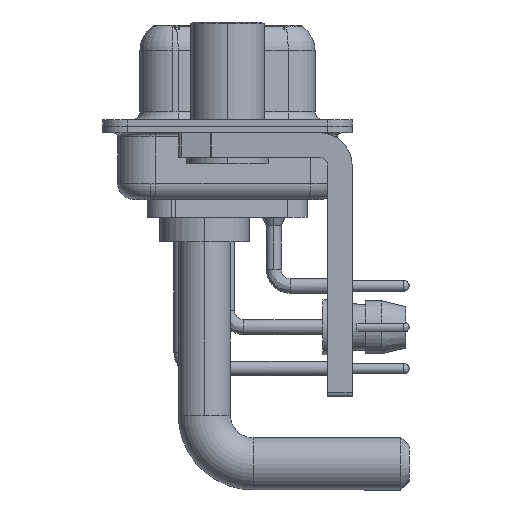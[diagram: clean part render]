
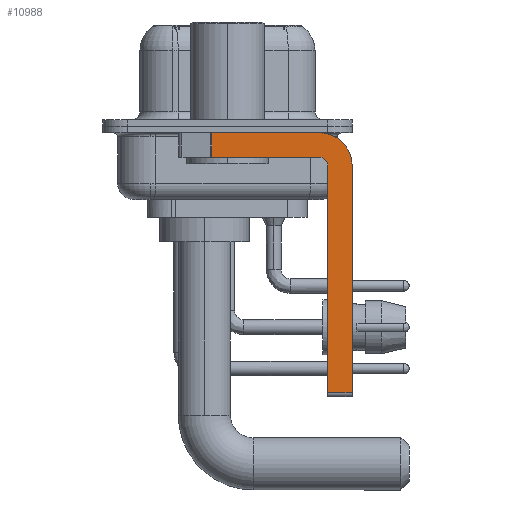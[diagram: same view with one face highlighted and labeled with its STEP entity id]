
A CAD part, left-side view. The second image highlights one B-rep face of the part: STEP entity #10988.
In plain terms, the highlighted planar face has unit normal (-1, 0, 0).
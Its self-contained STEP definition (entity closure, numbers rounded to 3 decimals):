
#671 = ORIENTED_EDGE ( 'NONE', *, *, #6378, .F. ) ;
#2028 = VECTOR ( 'NONE', #13443, 1000. ) ;
#2310 = CARTESIAN_POINT ( 'NONE',  ( -2.9, -5.65, -2.4 ) ) ;
#3599 = VERTEX_POINT ( 'NONE', #33242 ) ;
#4350 = VECTOR ( 'NONE', #29916, 1000. ) ;
#5146 = FACE_OUTER_BOUND ( 'NONE', #36842, .T. ) ;
#5217 = DIRECTION ( 'NONE',  ( 0., 1., 0. ) ) ;
#5401 = CARTESIAN_POINT ( 'NONE',  ( -2.9, -5.65, -1.9 ) ) ;
#6378 = EDGE_CURVE ( 'NONE', #30523, #20658, #31532, .T. ) ;
#6910 = AXIS2_PLACEMENT_3D ( 'NONE', #31079, #14211, #19491 ) ;
#7580 = VERTEX_POINT ( 'NONE', #15464 ) ;
#8199 = CARTESIAN_POINT ( 'NONE',  ( -2.9, -5.65, -2.4 ) ) ;
#9032 = CARTESIAN_POINT ( 'NONE',  ( -2.9, -7.65, -2.4 ) ) ;
#10414 = CARTESIAN_POINT ( 'NONE',  ( -2.9, -5.65, -16.35 ) ) ;
#10988 = ADVANCED_FACE ( 'NONE', ( #5146 ), #16698, .F. ) ;
#11016 = ORIENTED_EDGE ( 'NONE', *, *, #19971, .F. ) ;
#11122 = ORIENTED_EDGE ( 'NONE', *, *, #26427, .F. ) ;
#12929 = CARTESIAN_POINT ( 'NONE',  ( -2.9, -5.65, -0.4 ) ) ;
#12957 = CARTESIAN_POINT ( 'NONE',  ( -2.9, 3., -0.4 ) ) ;
#13041 = CARTESIAN_POINT ( 'NONE',  ( -2.9, 0.978, -1.9 ) ) ;
#13443 = DIRECTION ( 'NONE',  ( 0., -1., 0. ) ) ;
#13659 = VERTEX_POINT ( 'NONE', #28877 ) ;
#14211 = DIRECTION ( 'NONE',  ( -1., 0., 0. ) ) ;
#14961 = ORIENTED_EDGE ( 'NONE', *, *, #22165, .F. ) ;
#15464 = CARTESIAN_POINT ( 'NONE',  ( -2.9, 0.978, -1.9 ) ) ;
#16337 = LINE ( 'NONE', #28290, #29264 ) ;
#16340 = VECTOR ( 'NONE', #35541, 1000. ) ;
#16698 = PLANE ( 'NONE',  #20812 ) ;
#16909 = CARTESIAN_POINT ( 'NONE',  ( -2.9, -6.15, -16.6 ) ) ;
#16953 = LINE ( 'NONE', #5401, #28749 ) ;
#17800 = ORIENTED_EDGE ( 'NONE', *, *, #22647, .F. ) ;
#19280 = EDGE_CURVE ( 'NONE', #20658, #26713, #16337, .T. ) ;
#19332 = EDGE_CURVE ( 'NONE', #20355, #26713, #21759, .T. ) ;
#19491 = DIRECTION ( 'NONE',  ( 0., 0., 1. ) ) ;
#19744 = DIRECTION ( 'NONE',  ( 1., 0., 0. ) ) ;
#19971 = EDGE_CURVE ( 'NONE', #35182, #13659, #20223, .T. ) ;
#20223 = CIRCLE ( 'NONE', #6910, 0.5 ) ;
#20355 = VERTEX_POINT ( 'NONE', #21912 ) ;
#20658 = VERTEX_POINT ( 'NONE', #9032 ) ;
#20812 = AXIS2_PLACEMENT_3D ( 'NONE', #2310, #37004, #34530 ) ;
#21420 = CARTESIAN_POINT ( 'NONE',  ( -2.9, -6.15, -2.4 ) ) ;
#21759 = LINE ( 'NONE', #10414, #2028 ) ;
#21912 = CARTESIAN_POINT ( 'NONE',  ( -2.9, -6.15, -16.35 ) ) ;
#22165 = EDGE_CURVE ( 'NONE', #13659, #7580, #16953, .T. ) ;
#22460 = ORIENTED_EDGE ( 'NONE', *, *, #26897, .T. ) ;
#22647 = EDGE_CURVE ( 'NONE', #20355, #35182, #33988, .T. ) ;
#23932 = LINE ( 'NONE', #12957, #16340 ) ;
#24538 = VECTOR ( 'NONE', #31143, 1000. ) ;
#24767 = LINE ( 'NONE', #13041, #4350 ) ;
#25960 = ORIENTED_EDGE ( 'NONE', *, *, #19332, .T. ) ;
#26427 = EDGE_CURVE ( 'NONE', #3599, #30523, #23932, .T. ) ;
#26663 = ORIENTED_EDGE ( 'NONE', *, *, #19280, .F. ) ;
#26713 = VERTEX_POINT ( 'NONE', #35473 ) ;
#26897 = EDGE_CURVE ( 'NONE', #3599, #7580, #24767, .T. ) ;
#27899 = DIRECTION ( 'NONE',  ( 0., 0., -1. ) ) ;
#28290 = CARTESIAN_POINT ( 'NONE',  ( -2.9, -7.65, -2.4 ) ) ;
#28749 = VECTOR ( 'NONE', #5217, 1000. ) ;
#28877 = CARTESIAN_POINT ( 'NONE',  ( -2.9, -5.65, -1.9 ) ) ;
#29264 = VECTOR ( 'NONE', #27899, 1000. ) ;
#29916 = DIRECTION ( 'NONE',  ( 0., 0., -1. ) ) ;
#30523 = VERTEX_POINT ( 'NONE', #12929 ) ;
#31079 = CARTESIAN_POINT ( 'NONE',  ( -2.9, -5.65, -2.4 ) ) ;
#31143 = DIRECTION ( 'NONE',  ( 0., 0., 1. ) ) ;
#31335 = DIRECTION ( 'NONE',  ( 0., 0., -1. ) ) ;
#31532 = CIRCLE ( 'NONE', #33340, 2. ) ;
#33242 = CARTESIAN_POINT ( 'NONE',  ( -2.9, 0.978, -0.4 ) ) ;
#33340 = AXIS2_PLACEMENT_3D ( 'NONE', #8199, #19744, #31335 ) ;
#33988 = LINE ( 'NONE', #16909, #24538 ) ;
#34530 = DIRECTION ( 'NONE',  ( 0., 0., -1. ) ) ;
#35182 = VERTEX_POINT ( 'NONE', #21420 ) ;
#35473 = CARTESIAN_POINT ( 'NONE',  ( -2.9, -7.65, -16.35 ) ) ;
#35541 = DIRECTION ( 'NONE',  ( 0., -1., 0. ) ) ;
#36842 = EDGE_LOOP ( 'NONE', ( #11122, #22460, #14961, #11016, #17800, #25960, #26663, #671 ) ) ;
#37004 = DIRECTION ( 'NONE',  ( 1., 0., 0. ) ) ;
